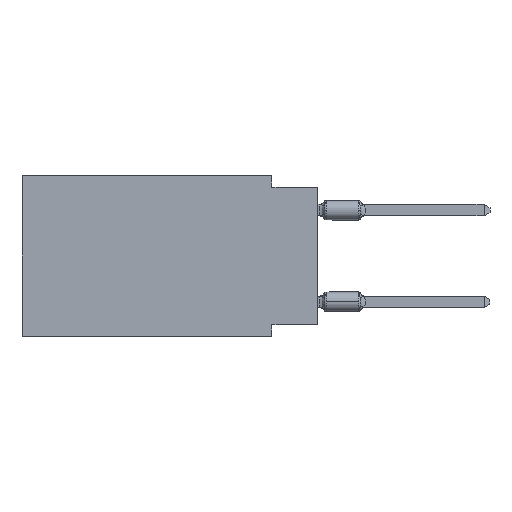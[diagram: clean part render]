
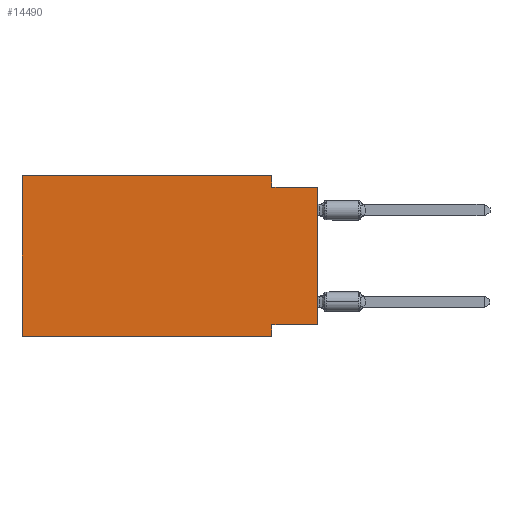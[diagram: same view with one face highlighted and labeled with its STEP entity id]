
A CAD part, left-side view. The second image highlights one B-rep face of the part: STEP entity #14490.
In plain terms, the highlighted planar face has unit normal (-1, 0, 0).
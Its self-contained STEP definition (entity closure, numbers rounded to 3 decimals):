
#190 = CARTESIAN_POINT ( 'NONE',  ( 0., 16.383, 0. ) ) ;
#627 = EDGE_CURVE ( 'NONE', #8050, #3602, #16599, .T. ) ;
#1296 = DIRECTION ( 'NONE',  ( 0., 0., -1. ) ) ;
#1300 = VERTEX_POINT ( 'NONE', #8493 ) ;
#1554 = VECTOR ( 'NONE', #10879, 1000. ) ;
#1690 = EDGE_CURVE ( 'NONE', #5471, #13120, #7370, .T. ) ;
#2144 = DIRECTION ( 'NONE',  ( 0., 0., -1. ) ) ;
#2300 = EDGE_CURVE ( 'NONE', #1300, #9574, #13961, .T. ) ;
#2507 = EDGE_CURVE ( 'NONE', #9149, #5471, #4199, .T. ) ;
#2664 = CARTESIAN_POINT ( 'NONE',  ( 0., 0., -0.635 ) ) ;
#2826 = DIRECTION ( 'NONE',  ( 0., 0., 1. ) ) ;
#2946 = CARTESIAN_POINT ( 'NONE',  ( 0., 0., -8.255 ) ) ;
#3113 = LINE ( 'NONE', #13638, #5815 ) ;
#3133 = CARTESIAN_POINT ( 'NONE',  ( 0., 0., -0.635 ) ) ;
#3268 = AXIS2_PLACEMENT_3D ( 'NONE', #14203, #4189, #1296 ) ;
#3602 = VERTEX_POINT ( 'NONE', #2664 ) ;
#3698 = DIRECTION ( 'NONE',  ( 0., 0., 1. ) ) ;
#3781 = VECTOR ( 'NONE', #9740, 1000. ) ;
#3782 = CARTESIAN_POINT ( 'NONE',  ( 0., 2.54, -8.89 ) ) ;
#4114 = ORIENTED_EDGE ( 'NONE', *, *, #12678, .F. ) ;
#4189 = DIRECTION ( 'NONE',  ( 1., 0., 0. ) ) ;
#4199 = LINE ( 'NONE', #190, #13009 ) ;
#4512 = EDGE_CURVE ( 'NONE', #13120, #10082, #9187, .T. ) ;
#4881 = ORIENTED_EDGE ( 'NONE', *, *, #2507, .F. ) ;
#5029 = EDGE_CURVE ( 'NONE', #9149, #9574, #3113, .T. ) ;
#5436 = DIRECTION ( 'NONE',  ( 0., -1., 0. ) ) ;
#5471 = VERTEX_POINT ( 'NONE', #6377 ) ;
#5815 = VECTOR ( 'NONE', #6953, 1000. ) ;
#6318 = CARTESIAN_POINT ( 'NONE',  ( 0., 2.54, -8.89 ) ) ;
#6377 = CARTESIAN_POINT ( 'NONE',  ( 0., 16.383, 0. ) ) ;
#6932 = ORIENTED_EDGE ( 'NONE', *, *, #4512, .F. ) ;
#6953 = DIRECTION ( 'NONE',  ( 0., -1., 0. ) ) ;
#7370 = LINE ( 'NONE', #9824, #3781 ) ;
#8050 = VERTEX_POINT ( 'NONE', #2946 ) ;
#8493 = CARTESIAN_POINT ( 'NONE',  ( 0., 2.54, -8.255 ) ) ;
#9039 = FACE_OUTER_BOUND ( 'NONE', #15989, .T. ) ;
#9149 = VERTEX_POINT ( 'NONE', #9158 ) ;
#9158 = CARTESIAN_POINT ( 'NONE',  ( 0., 16.383, -8.89 ) ) ;
#9187 = LINE ( 'NONE', #10776, #16370 ) ;
#9567 = ORIENTED_EDGE ( 'NONE', *, *, #5029, .T. ) ;
#9574 = VERTEX_POINT ( 'NONE', #3782 ) ;
#9740 = DIRECTION ( 'NONE',  ( 0., -1., 0. ) ) ;
#9748 = VECTOR ( 'NONE', #2144, 1000. ) ;
#9824 = CARTESIAN_POINT ( 'NONE',  ( 0., 16.383, 0. ) ) ;
#9842 = ORIENTED_EDGE ( 'NONE', *, *, #1690, .F. ) ;
#10082 = VERTEX_POINT ( 'NONE', #14534 ) ;
#10149 = EDGE_CURVE ( 'NONE', #8050, #1300, #10956, .T. ) ;
#10776 = CARTESIAN_POINT ( 'NONE',  ( 0., 2.54, 0. ) ) ;
#10862 = LINE ( 'NONE', #3133, #13744 ) ;
#10879 = DIRECTION ( 'NONE',  ( 0., 1., 0. ) ) ;
#10956 = LINE ( 'NONE', #12322, #1554 ) ;
#11623 = ORIENTED_EDGE ( 'NONE', *, *, #2300, .F. ) ;
#11908 = PLANE ( 'NONE',  #3268 ) ;
#12322 = CARTESIAN_POINT ( 'NONE',  ( 0., 0., -8.255 ) ) ;
#12678 = EDGE_CURVE ( 'NONE', #10082, #3602, #10862, .T. ) ;
#13009 = VECTOR ( 'NONE', #2826, 1000. ) ;
#13120 = VERTEX_POINT ( 'NONE', #14503 ) ;
#13638 = CARTESIAN_POINT ( 'NONE',  ( 0., 16.383, -8.89 ) ) ;
#13744 = VECTOR ( 'NONE', #5436, 1000. ) ;
#13961 = LINE ( 'NONE', #6318, #9748 ) ;
#14062 = VECTOR ( 'NONE', #3698, 1000. ) ;
#14203 = CARTESIAN_POINT ( 'NONE',  ( 0., 16.383, 0. ) ) ;
#14490 = ADVANCED_FACE ( 'NONE', ( #9039 ), #11908, .F. ) ;
#14503 = CARTESIAN_POINT ( 'NONE',  ( 0., 2.54, 0. ) ) ;
#14534 = CARTESIAN_POINT ( 'NONE',  ( 0., 2.54, -0.635 ) ) ;
#14899 = ORIENTED_EDGE ( 'NONE', *, *, #10149, .F. ) ;
#15330 = CARTESIAN_POINT ( 'NONE',  ( 0., 0., 0. ) ) ;
#15989 = EDGE_LOOP ( 'NONE', ( #16648, #4114, #6932, #9842, #4881, #9567, #11623, #14899 ) ) ;
#16048 = DIRECTION ( 'NONE',  ( 0., 0., -1. ) ) ;
#16370 = VECTOR ( 'NONE', #16048, 1000. ) ;
#16599 = LINE ( 'NONE', #15330, #14062 ) ;
#16648 = ORIENTED_EDGE ( 'NONE', *, *, #627, .T. ) ;
